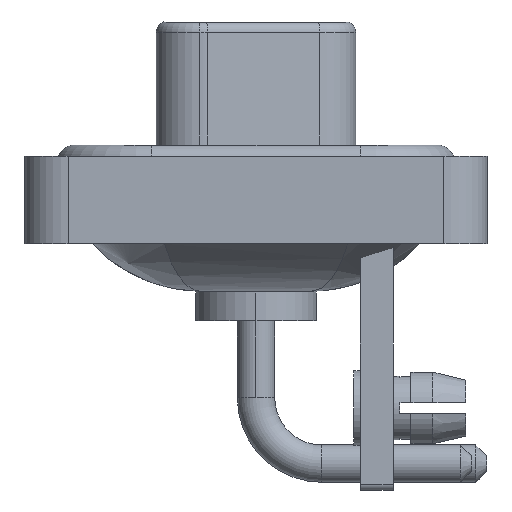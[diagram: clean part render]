
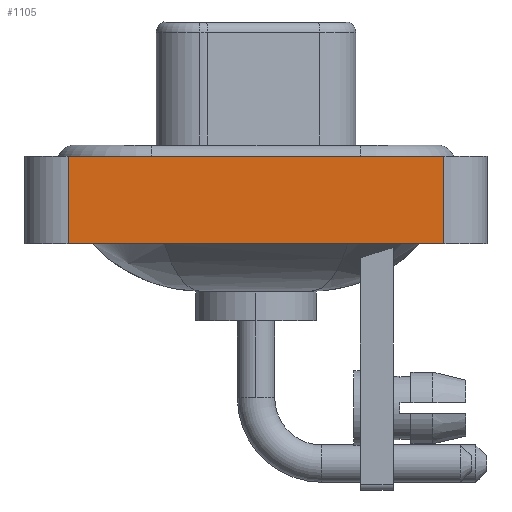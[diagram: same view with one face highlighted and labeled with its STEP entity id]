
A CAD part, left-side view. The second image highlights one B-rep face of the part: STEP entity #1105.
In plain terms, the highlighted planar face has unit normal (-1, 0, 0).
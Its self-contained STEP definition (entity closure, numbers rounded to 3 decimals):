
#1105 = ADVANCED_FACE ( 'NONE', ( #17039 ), #19813, .T. ) ;
#1236 = VERTEX_POINT ( 'NONE', #7673 ) ;
#1257 = EDGE_CURVE ( 'NONE', #16135, #5436, #10860, .T. ) ;
#1763 = EDGE_CURVE ( 'NONE', #1236, #17330, #14468, .T. ) ;
#2759 = CARTESIAN_POINT ( 'NONE',  ( -7.3, -8.55, 0.4 ) ) ;
#3526 = DIRECTION ( 'NONE',  ( 0., 0., 1. ) ) ;
#3615 = VECTOR ( 'NONE', #5387, 1000. ) ;
#3667 = CARTESIAN_POINT ( 'NONE',  ( -7.3, 8.55, -3.6 ) ) ;
#4347 = VECTOR ( 'NONE', #3526, 1000. ) ;
#4715 = DIRECTION ( 'NONE',  ( 0., -1., 0. ) ) ;
#5314 = VECTOR ( 'NONE', #5618, 1000. ) ;
#5387 = DIRECTION ( 'NONE',  ( 0., 0., 1. ) ) ;
#5436 = VERTEX_POINT ( 'NONE', #8419 ) ;
#5501 = CARTESIAN_POINT ( 'NONE',  ( -7.3, 8.55, -3.6 ) ) ;
#5583 = VECTOR ( 'NONE', #4715, 1000. ) ;
#5618 = DIRECTION ( 'NONE',  ( 0., -1., 0. ) ) ;
#7673 = CARTESIAN_POINT ( 'NONE',  ( -7.3, 8.55, 0.4 ) ) ;
#8088 = AXIS2_PLACEMENT_3D ( 'NONE', #15616, #13111, #18873 ) ;
#8196 = CARTESIAN_POINT ( 'NONE',  ( -7.3, -8.55, 0.4 ) ) ;
#8419 = CARTESIAN_POINT ( 'NONE',  ( -7.3, -8.55, -3.6 ) ) ;
#10513 = LINE ( 'NONE', #5501, #3615 ) ;
#10860 = LINE ( 'NONE', #20632, #5314 ) ;
#11840 = EDGE_CURVE ( 'NONE', #5436, #17330, #16908, .T. ) ;
#13111 = DIRECTION ( 'NONE',  ( -1., 0., 0. ) ) ;
#13602 = EDGE_LOOP ( 'NONE', ( #20274, #20480, #17451, #21509 ) ) ;
#14468 = LINE ( 'NONE', #8196, #5583 ) ;
#15616 = CARTESIAN_POINT ( 'NONE',  ( -7.3, -8.55, -3.6 ) ) ;
#16135 = VERTEX_POINT ( 'NONE', #3667 ) ;
#16908 = LINE ( 'NONE', #18337, #4347 ) ;
#17039 = FACE_OUTER_BOUND ( 'NONE', #13602, .T. ) ;
#17330 = VERTEX_POINT ( 'NONE', #2759 ) ;
#17451 = ORIENTED_EDGE ( 'NONE', *, *, #20827, .F. ) ;
#18337 = CARTESIAN_POINT ( 'NONE',  ( -7.3, -8.55, -3.6 ) ) ;
#18873 = DIRECTION ( 'NONE',  ( 0., 0., 1. ) ) ;
#19813 = PLANE ( 'NONE',  #8088 ) ;
#20274 = ORIENTED_EDGE ( 'NONE', *, *, #11840, .T. ) ;
#20480 = ORIENTED_EDGE ( 'NONE', *, *, #1763, .F. ) ;
#20632 = CARTESIAN_POINT ( 'NONE',  ( -7.3, -8.55, -3.6 ) ) ;
#20827 = EDGE_CURVE ( 'NONE', #16135, #1236, #10513, .T. ) ;
#21509 = ORIENTED_EDGE ( 'NONE', *, *, #1257, .T. ) ;
